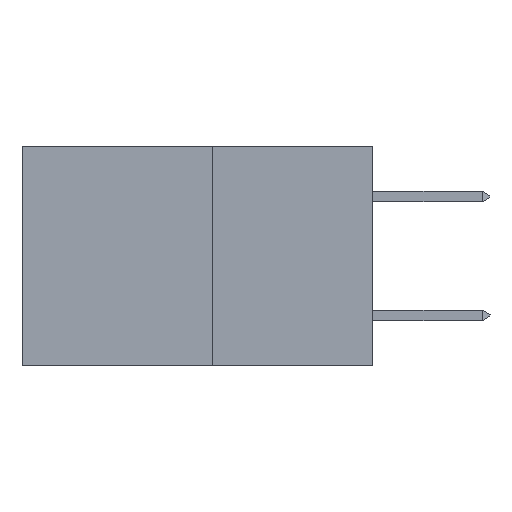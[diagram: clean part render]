
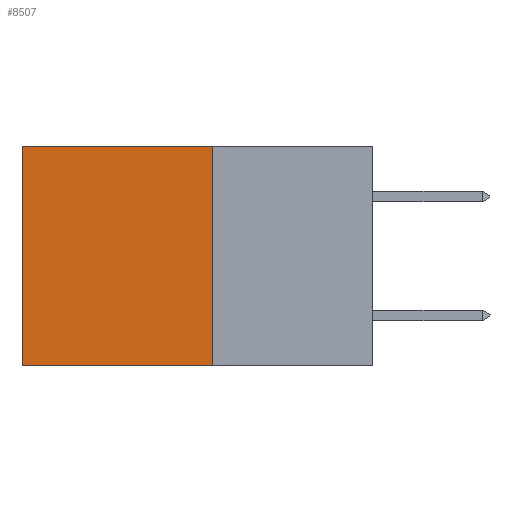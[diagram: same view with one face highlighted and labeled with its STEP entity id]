
A CAD part, left-side view. The second image highlights one B-rep face of the part: STEP entity #8507.
In plain terms, the highlighted planar face has unit normal (-1, 0, 0).
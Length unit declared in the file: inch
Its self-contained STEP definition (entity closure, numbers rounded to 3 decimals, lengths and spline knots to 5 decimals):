
#110 = CARTESIAN_POINT ( 'NONE',  ( 0.277, 0.27, -0.37 ) ) ;
#1144 = ORIENTED_EDGE ( 'NONE', *, *, #28696, .F. ) ;
#1438 = CARTESIAN_POINT ( 'NONE',  ( 0.277, 0.27, -0.37 ) ) ;
#2165 = LINE ( 'NONE', #110, #28439 ) ;
#2192 = LINE ( 'NONE', #19991, #16425 ) ;
#2837 = CARTESIAN_POINT ( 'NONE',  ( 0.277, 0.59, -0.37 ) ) ;
#4290 = CARTESIAN_POINT ( 'NONE',  ( 0.277, 0.59, -0.37 ) ) ;
#4748 = LINE ( 'NONE', #10595, #12636 ) ;
#4782 = CARTESIAN_POINT ( 'NONE',  ( 0.277, 0.27, -0.37 ) ) ;
#4936 = EDGE_LOOP ( 'NONE', ( #11150, #1144, #16814, #10479 ) ) ;
#6386 = LINE ( 'NONE', #4290, #14455 ) ;
#7682 = EDGE_CURVE ( 'NONE', #10554, #25206, #6386, .T. ) ;
#8507 = ADVANCED_FACE ( 'NONE', ( #26597 ), #23878, .F. ) ;
#9542 = VERTEX_POINT ( 'NONE', #22933 ) ;
#9665 = DIRECTION ( 'NONE',  ( 1., 0., 0. ) ) ;
#10479 = ORIENTED_EDGE ( 'NONE', *, *, #29617, .T. ) ;
#10554 = VERTEX_POINT ( 'NONE', #28755 ) ;
#10595 = CARTESIAN_POINT ( 'NONE',  ( 0.277, 0.27, 0. ) ) ;
#11150 = ORIENTED_EDGE ( 'NONE', *, *, #7682, .T. ) ;
#12636 = VECTOR ( 'NONE', #15326, 39.37008 ) ;
#12921 = DIRECTION ( 'NONE',  ( 0., 0., -1. ) ) ;
#14455 = VECTOR ( 'NONE', #18495, 39.37008 ) ;
#15326 = DIRECTION ( 'NONE',  ( 0., 1., 0. ) ) ;
#16425 = VECTOR ( 'NONE', #12921, 39.37008 ) ;
#16621 = AXIS2_PLACEMENT_3D ( 'NONE', #4782, #9665, #26259 ) ;
#16814 = ORIENTED_EDGE ( 'NONE', *, *, #28211, .F. ) ;
#16950 = DIRECTION ( 'NONE',  ( 0., 1., 0. ) ) ;
#18495 = DIRECTION ( 'NONE',  ( 0., 0., -1. ) ) ;
#19991 = CARTESIAN_POINT ( 'NONE',  ( 0.277, 0.27, -0.37 ) ) ;
#21533 = VERTEX_POINT ( 'NONE', #1438 ) ;
#22933 = CARTESIAN_POINT ( 'NONE',  ( 0.277, 0.27, 0. ) ) ;
#23878 = PLANE ( 'NONE',  #16621 ) ;
#25206 = VERTEX_POINT ( 'NONE', #2837 ) ;
#26259 = DIRECTION ( 'NONE',  ( 0., 0., -1. ) ) ;
#26597 = FACE_OUTER_BOUND ( 'NONE', #4936, .T. ) ;
#28211 = EDGE_CURVE ( 'NONE', #9542, #21533, #2192, .T. ) ;
#28439 = VECTOR ( 'NONE', #16950, 39.37008 ) ;
#28696 = EDGE_CURVE ( 'NONE', #21533, #25206, #2165, .T. ) ;
#28755 = CARTESIAN_POINT ( 'NONE',  ( 0.277, 0.59, 0. ) ) ;
#29617 = EDGE_CURVE ( 'NONE', #9542, #10554, #4748, .T. ) ;
